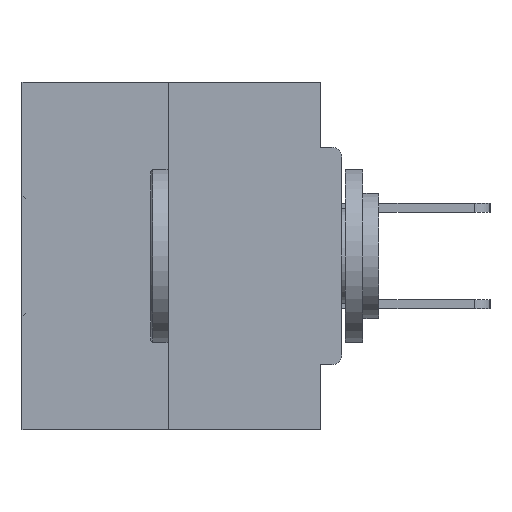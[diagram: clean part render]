
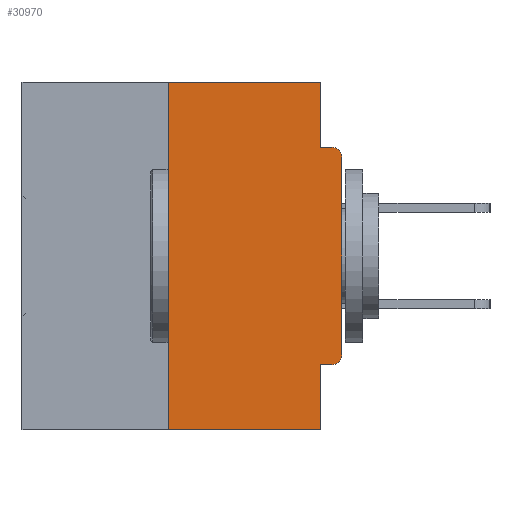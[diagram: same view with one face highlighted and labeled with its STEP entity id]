
A CAD part, left-side view. The second image highlights one B-rep face of the part: STEP entity #30970.
In plain terms, the highlighted planar face has unit normal (-1, 0, 0).
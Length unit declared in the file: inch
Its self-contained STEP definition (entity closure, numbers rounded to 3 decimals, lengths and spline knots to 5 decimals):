
#1370 = EDGE_CURVE ( 'NONE', #35021, #1945, #24474, .T. ) ;
#1396 = ORIENTED_EDGE ( 'NONE', *, *, #22784, .F. ) ;
#1813 = AXIS2_PLACEMENT_3D ( 'NONE', #39158, #42379, #42656 ) ;
#1945 = VERTEX_POINT ( 'NONE', #2411 ) ;
#2086 = CARTESIAN_POINT ( 'NONE',  ( 0., 0.25, -0.5 ) ) ;
#2185 = VERTEX_POINT ( 'NONE', #7063 ) ;
#2235 = DIRECTION ( 'NONE',  ( 0., -1., 0. ) ) ;
#2411 = CARTESIAN_POINT ( 'NONE',  ( 0., 0., -0.3915 ) ) ;
#2919 = DIRECTION ( 'NONE',  ( 0., 0., -1. ) ) ;
#4291 = VERTEX_POINT ( 'NONE', #43389 ) ;
#4354 = ORIENTED_EDGE ( 'NONE', *, *, #1370, .T. ) ;
#4835 = VECTOR ( 'NONE', #28741, 39.37008 ) ;
#5077 = CARTESIAN_POINT ( 'NONE',  ( 0., 0.031, -0.5 ) ) ;
#5288 = PLANE ( 'NONE',  #14083 ) ;
#5374 = DIRECTION ( 'NONE',  ( 0., 0., -1. ) ) ;
#5407 = DIRECTION ( 'NONE',  ( -1., 0., 0. ) ) ;
#6034 = VECTOR ( 'NONE', #33032, 39.37008 ) ;
#6208 = VECTOR ( 'NONE', #2235, 39.37008 ) ;
#7063 = CARTESIAN_POINT ( 'NONE',  ( 0., 0.031, -0.4065 ) ) ;
#7895 = ORIENTED_EDGE ( 'NONE', *, *, #16240, .T. ) ;
#8011 = VECTOR ( 'NONE', #20051, 39.37008 ) ;
#8307 = VECTOR ( 'NONE', #5374, 39.37008 ) ;
#8789 = VECTOR ( 'NONE', #24129, 39.37008 ) ;
#8892 = FACE_OUTER_BOUND ( 'NONE', #30006, .T. ) ;
#8954 = CARTESIAN_POINT ( 'NONE',  ( 0., 0.46, 0. ) ) ;
#8994 = DIRECTION ( 'NONE',  ( 0., 0., 1. ) ) ;
#9060 = CARTESIAN_POINT ( 'NONE',  ( 0., 0.031, -0.0935 ) ) ;
#9379 = LINE ( 'NONE', #19011, #6208 ) ;
#9521 = EDGE_CURVE ( 'NONE', #24853, #27344, #9379, .T. ) ;
#9561 = LINE ( 'NONE', #11686, #4835 ) ;
#10935 = LINE ( 'NONE', #39582, #8307 ) ;
#11686 = CARTESIAN_POINT ( 'NONE',  ( 0., 0., 0. ) ) ;
#12296 = ORIENTED_EDGE ( 'NONE', *, *, #20107, .F. ) ;
#14083 = AXIS2_PLACEMENT_3D ( 'NONE', #8954, #22493, #25895 ) ;
#15452 = CARTESIAN_POINT ( 'NONE',  ( 0., 0.25, 0. ) ) ;
#16240 = EDGE_CURVE ( 'NONE', #1945, #4291, #9561, .T. ) ;
#16520 = ORIENTED_EDGE ( 'NONE', *, *, #35642, .T. ) ;
#16762 = CARTESIAN_POINT ( 'NONE',  ( 0., 0.015, -0.4065 ) ) ;
#19011 = CARTESIAN_POINT ( 'NONE',  ( 0., 0., -0.0935 ) ) ;
#19331 = VERTEX_POINT ( 'NONE', #15452 ) ;
#19697 = CARTESIAN_POINT ( 'NONE',  ( 0., 0.031, 0. ) ) ;
#20051 = DIRECTION ( 'NONE',  ( 0., 1., 0. ) ) ;
#20107 = EDGE_CURVE ( 'NONE', #35021, #2185, #34337, .T. ) ;
#22493 = DIRECTION ( 'NONE',  ( 1., 0., 0. ) ) ;
#22784 = EDGE_CURVE ( 'NONE', #36602, #19331, #34047, .T. ) ;
#22839 = ORIENTED_EDGE ( 'NONE', *, *, #26013, .T. ) ;
#23315 = VERTEX_POINT ( 'NONE', #19697 ) ;
#24129 = DIRECTION ( 'NONE',  ( 0., -1., 0. ) ) ;
#24474 = CIRCLE ( 'NONE', #33698, 0.015 ) ;
#24853 = VERTEX_POINT ( 'NONE', #9060 ) ;
#25436 = EDGE_CURVE ( 'NONE', #23315, #24853, #34599, .T. ) ;
#25441 = EDGE_CURVE ( 'NONE', #2185, #40196, #10935, .T. ) ;
#25507 = EDGE_CURVE ( 'NONE', #19331, #23315, #43456, .T. ) ;
#25690 = DIRECTION ( 'NONE',  ( 0., 0., -1. ) ) ;
#25726 = CARTESIAN_POINT ( 'NONE',  ( 0., 0.015, -0.3915 ) ) ;
#25895 = DIRECTION ( 'NONE',  ( 0., 0., -1. ) ) ;
#26013 = EDGE_CURVE ( 'NONE', #4291, #27344, #26697, .T. ) ;
#26697 = CIRCLE ( 'NONE', #1813, 0.015 ) ;
#26730 = CARTESIAN_POINT ( 'NONE',  ( 0., 0.46, -0.5 ) ) ;
#27344 = VERTEX_POINT ( 'NONE', #27552 ) ;
#27552 = CARTESIAN_POINT ( 'NONE',  ( 0., 0.015, -0.0935 ) ) ;
#28741 = DIRECTION ( 'NONE',  ( 0., 0., 1. ) ) ;
#29106 = ORIENTED_EDGE ( 'NONE', *, *, #9521, .F. ) ;
#29487 = CARTESIAN_POINT ( 'NONE',  ( 0., 0.031, 0. ) ) ;
#29731 = CARTESIAN_POINT ( 'NONE',  ( 0., 0.25, 0. ) ) ;
#30006 = EDGE_LOOP ( 'NONE', ( #31160, #1396, #16520, #36310, #12296, #4354, #7895, #22839, #29106, #39572 ) ) ;
#30970 = ADVANCED_FACE ( 'NONE', ( #8892 ), #5288, .F. ) ;
#31160 = ORIENTED_EDGE ( 'NONE', *, *, #25507, .F. ) ;
#33032 = DIRECTION ( 'NONE',  ( 0., -1., 0. ) ) ;
#33558 = CARTESIAN_POINT ( 'NONE',  ( 0., 0., -0.4065 ) ) ;
#33698 = AXIS2_PLACEMENT_3D ( 'NONE', #25726, #5407, #2919 ) ;
#34047 = LINE ( 'NONE', #29731, #37680 ) ;
#34301 = CARTESIAN_POINT ( 'NONE',  ( 0., 0.46, 0. ) ) ;
#34337 = LINE ( 'NONE', #33558, #8011 ) ;
#34599 = LINE ( 'NONE', #29487, #39806 ) ;
#35021 = VERTEX_POINT ( 'NONE', #16762 ) ;
#35642 = EDGE_CURVE ( 'NONE', #36602, #40196, #42797, .T. ) ;
#36310 = ORIENTED_EDGE ( 'NONE', *, *, #25441, .F. ) ;
#36602 = VERTEX_POINT ( 'NONE', #2086 ) ;
#37680 = VECTOR ( 'NONE', #8994, 39.37008 ) ;
#39158 = CARTESIAN_POINT ( 'NONE',  ( 0., 0.015, -0.1085 ) ) ;
#39572 = ORIENTED_EDGE ( 'NONE', *, *, #25436, .F. ) ;
#39582 = CARTESIAN_POINT ( 'NONE',  ( 0., 0.031, -0.5 ) ) ;
#39806 = VECTOR ( 'NONE', #25690, 39.37008 ) ;
#40196 = VERTEX_POINT ( 'NONE', #5077 ) ;
#42379 = DIRECTION ( 'NONE',  ( -1., 0., 0. ) ) ;
#42656 = DIRECTION ( 'NONE',  ( 0., 0., -1. ) ) ;
#42797 = LINE ( 'NONE', #26730, #6034 ) ;
#43389 = CARTESIAN_POINT ( 'NONE',  ( 0., 0., -0.1085 ) ) ;
#43456 = LINE ( 'NONE', #34301, #8789 ) ;
